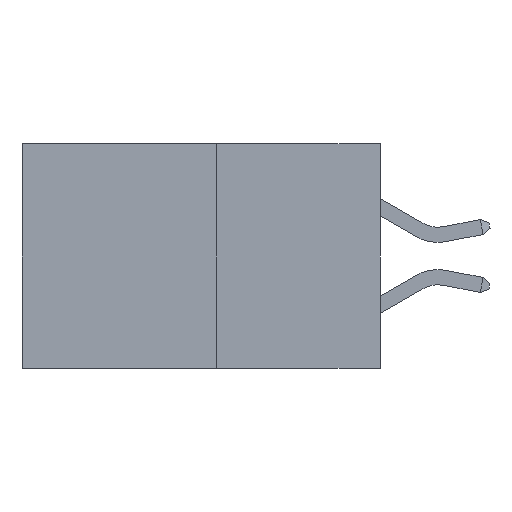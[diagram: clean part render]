
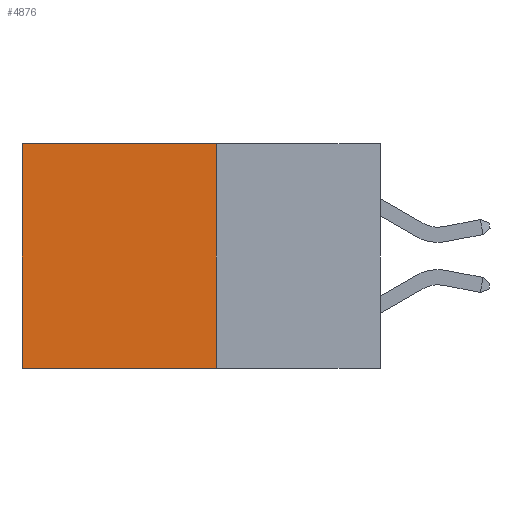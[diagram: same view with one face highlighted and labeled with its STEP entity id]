
A CAD part, left-side view. The second image highlights one B-rep face of the part: STEP entity #4876.
In plain terms, the highlighted planar face has unit normal (-1, 0, 0).
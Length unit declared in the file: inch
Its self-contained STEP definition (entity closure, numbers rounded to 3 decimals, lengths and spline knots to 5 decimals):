
#1051 = VECTOR ( 'NONE', #13224, 39.37008 ) ;
#2392 = EDGE_CURVE ( 'NONE', #14456, #7884, #21521, .T. ) ;
#2681 = VECTOR ( 'NONE', #11444, 39.37008 ) ;
#3190 = FACE_OUTER_BOUND ( 'NONE', #4304, .T. ) ;
#3906 = EDGE_CURVE ( 'NONE', #7884, #11512, #18927, .T. ) ;
#4304 = EDGE_LOOP ( 'NONE', ( #21214, #17943, #5692, #10588 ) ) ;
#4422 = VECTOR ( 'NONE', #19791, 39.37008 ) ;
#4583 = LINE ( 'NONE', #8997, #8506 ) ;
#4876 = ADVANCED_FACE ( 'NONE', ( #3190 ), #18233, .F. ) ;
#5692 = ORIENTED_EDGE ( 'NONE', *, *, #2392, .F. ) ;
#6949 = EDGE_CURVE ( 'NONE', #14456, #9267, #15576, .T. ) ;
#7028 = EDGE_CURVE ( 'NONE', #9267, #11512, #4583, .T. ) ;
#7884 = VERTEX_POINT ( 'NONE', #14643 ) ;
#8506 = VECTOR ( 'NONE', #9140, 39.37008 ) ;
#8997 = CARTESIAN_POINT ( 'NONE',  ( 0.277, 0.59, -0.37 ) ) ;
#9140 = DIRECTION ( 'NONE',  ( 0., 0., -1. ) ) ;
#9267 = VERTEX_POINT ( 'NONE', #13754 ) ;
#10588 = ORIENTED_EDGE ( 'NONE', *, *, #6949, .T. ) ;
#11444 = DIRECTION ( 'NONE',  ( 0., 1., 0. ) ) ;
#11500 = CARTESIAN_POINT ( 'NONE',  ( 0.277, 0.27, 0. ) ) ;
#11512 = VERTEX_POINT ( 'NONE', #18310 ) ;
#12500 = CARTESIAN_POINT ( 'NONE',  ( 0.277, 0.27, -0.37 ) ) ;
#12842 = AXIS2_PLACEMENT_3D ( 'NONE', #17886, #17862, #17857 ) ;
#13224 = DIRECTION ( 'NONE',  ( 0., 1., 0. ) ) ;
#13754 = CARTESIAN_POINT ( 'NONE',  ( 0.277, 0.59, 0. ) ) ;
#14456 = VERTEX_POINT ( 'NONE', #14570 ) ;
#14570 = CARTESIAN_POINT ( 'NONE',  ( 0.277, 0.27, 0. ) ) ;
#14643 = CARTESIAN_POINT ( 'NONE',  ( 0.277, 0.27, -0.37 ) ) ;
#15506 = CARTESIAN_POINT ( 'NONE',  ( 0.277, 0.27, -0.37 ) ) ;
#15576 = LINE ( 'NONE', #11500, #2681 ) ;
#17857 = DIRECTION ( 'NONE',  ( 0., 0., -1. ) ) ;
#17862 = DIRECTION ( 'NONE',  ( 1., 0., 0. ) ) ;
#17886 = CARTESIAN_POINT ( 'NONE',  ( 0.277, 0.27, -0.37 ) ) ;
#17943 = ORIENTED_EDGE ( 'NONE', *, *, #3906, .F. ) ;
#18233 = PLANE ( 'NONE',  #12842 ) ;
#18310 = CARTESIAN_POINT ( 'NONE',  ( 0.277, 0.59, -0.37 ) ) ;
#18927 = LINE ( 'NONE', #12500, #1051 ) ;
#19791 = DIRECTION ( 'NONE',  ( 0., 0., -1. ) ) ;
#21214 = ORIENTED_EDGE ( 'NONE', *, *, #7028, .T. ) ;
#21521 = LINE ( 'NONE', #15506, #4422 ) ;
